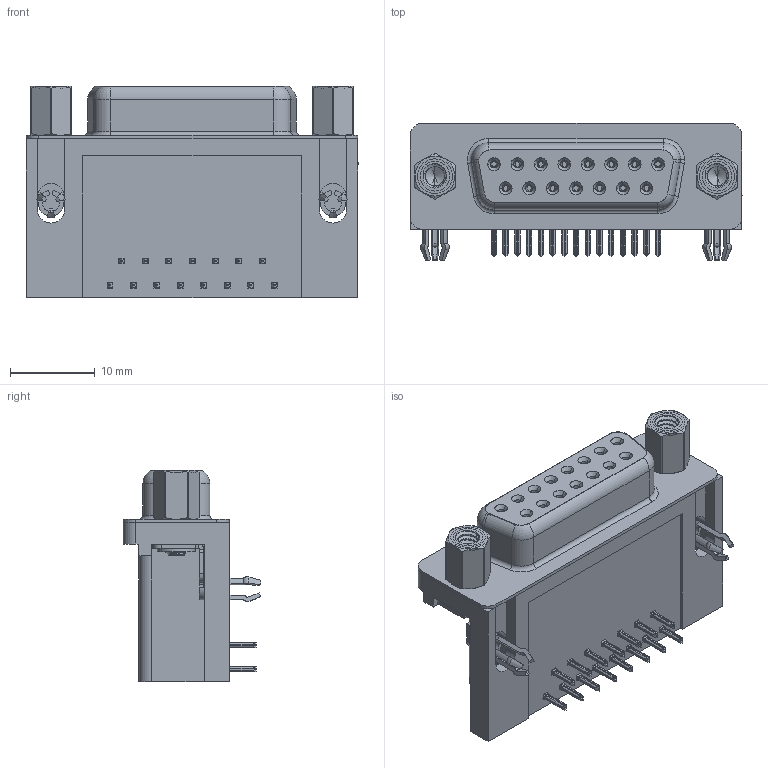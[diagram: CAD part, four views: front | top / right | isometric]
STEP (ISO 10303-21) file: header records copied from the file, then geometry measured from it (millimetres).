
FILE_DESCRIPTION (( 'STEP AP203' ), '1' );
FILE_NAME ('626-015-262-043.STEP', '2018-11-07T00:20:57', ( '' ), ( '' ), 'SwSTEP 2.0', 'SolidWorks 2016', '' );
FILE_SCHEMA (( 'CONFIG_CONTROL_DESIGN' ));
Length unit declared in the file: millimetre
Products named in the file (8): 626 Housing_15 Socket; 626 Shell_15 Socket; 626 Contact Bottom; 626 Contact Top; 626 3 Prong Board Lock; 626 Round Threaded Standoff; 626 4-40 Hex Standoff 5; 626-015-262-043
Assembly tree (23 placements, depth 2):
  626-015-262-043
    626 Housing_15 Socket
    626 Shell_15 Socket
    626 Contact Bottom  x7
    626 Contact Top  x8
    626 3 Prong Board Lock  x2
    626 Round Threaded Standoff  x2
    626 4-40 Hex Standoff 5  x2
Bounding box: 39.22 x 16.25 x 24.96 mm (x, y, z)
Volume: 7556.3 mm3; surface area: 8772.5 mm2
Topology: 23 solids, 23 shells, 2649 faces, 7020 edges, 4430 vertices
Faces by surface type: plane 1124, cylinder 691, bspline 540, cone 248, torus 46
Entity records: 33104 total; most frequent: CARTESIAN_POINT 12725, ORIENTED_EDGE 4182, DIRECTION 3669, EDGE_CURVE 2091, VERTEX_POINT 1341, AXIS2_PLACEMENT_3D 1231, VECTOR 1207, LINE 1207
